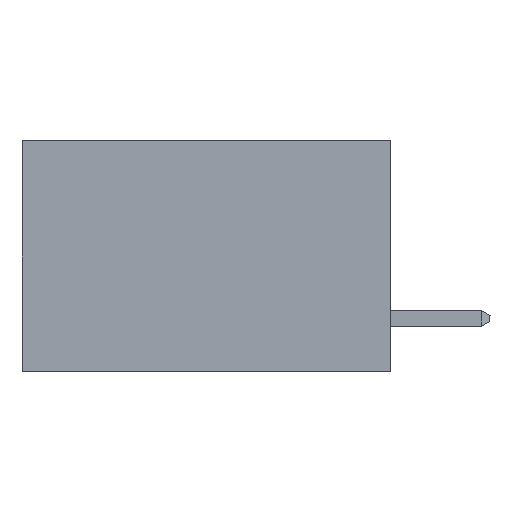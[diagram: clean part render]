
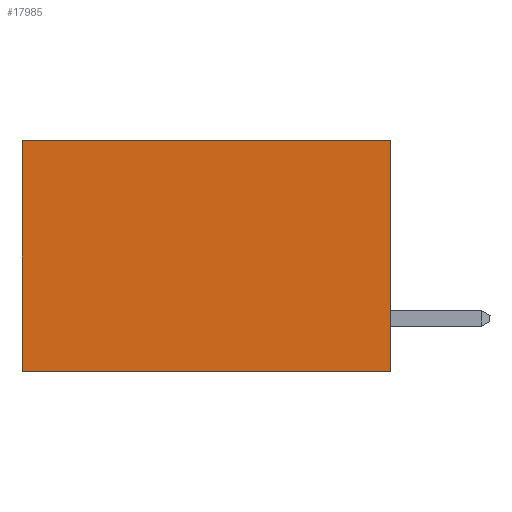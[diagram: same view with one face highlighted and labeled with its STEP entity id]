
A CAD part, left-side view. The second image highlights one B-rep face of the part: STEP entity #17985.
In plain terms, the highlighted planar face has unit normal (-1, 0, 0).
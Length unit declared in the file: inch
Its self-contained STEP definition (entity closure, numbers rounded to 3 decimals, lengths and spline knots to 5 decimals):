
#2036 = VERTEX_POINT ( 'NONE', #12464 ) ;
#2670 = EDGE_CURVE ( 'NONE', #18537, #3375, #8628, .T. ) ;
#3125 = AXIS2_PLACEMENT_3D ( 'NONE', #4354, #16279, #7392 ) ;
#3375 = VERTEX_POINT ( 'NONE', #13923 ) ;
#4354 = CARTESIAN_POINT ( 'NONE',  ( 0.277, 0., -0.37 ) ) ;
#4413 = PLANE ( 'NONE',  #3125 ) ;
#4489 = VERTEX_POINT ( 'NONE', #13480 ) ;
#4725 = DIRECTION ( 'NONE',  ( 0., 1., 0. ) ) ;
#4790 = VECTOR ( 'NONE', #13494, 39.37008 ) ;
#4847 = EDGE_CURVE ( 'NONE', #2036, #18537, #18902, .T. ) ;
#4871 = ORIENTED_EDGE ( 'NONE', *, *, #6501, .T. ) ;
#5317 = ORIENTED_EDGE ( 'NONE', *, *, #2670, .F. ) ;
#5808 = ORIENTED_EDGE ( 'NONE', *, *, #4847, .F. ) ;
#6067 = EDGE_LOOP ( 'NONE', ( #8196, #5317, #5808, #4871 ) ) ;
#6172 = LINE ( 'NONE', #13827, #4790 ) ;
#6501 = EDGE_CURVE ( 'NONE', #2036, #4489, #6172, .T. ) ;
#7392 = DIRECTION ( 'NONE',  ( 0., 0., -1. ) ) ;
#8167 = VECTOR ( 'NONE', #4725, 39.37008 ) ;
#8196 = ORIENTED_EDGE ( 'NONE', *, *, #14870, .T. ) ;
#8628 = LINE ( 'NONE', #17657, #8167 ) ;
#9698 = CARTESIAN_POINT ( 'NONE',  ( 0.277, 0., -0.37 ) ) ;
#9716 = DIRECTION ( 'NONE',  ( 0., 0., -1. ) ) ;
#10768 = FACE_OUTER_BOUND ( 'NONE', #6067, .T. ) ;
#11410 = VECTOR ( 'NONE', #9716, 39.37008 ) ;
#12464 = CARTESIAN_POINT ( 'NONE',  ( 0.277, 0., 0. ) ) ;
#12787 = VECTOR ( 'NONE', #17960, 39.37008 ) ;
#13095 = CARTESIAN_POINT ( 'NONE',  ( 0.277, 0., -0.37 ) ) ;
#13480 = CARTESIAN_POINT ( 'NONE',  ( 0.277, 0.59, 0. ) ) ;
#13494 = DIRECTION ( 'NONE',  ( 0., 1., 0. ) ) ;
#13827 = CARTESIAN_POINT ( 'NONE',  ( 0.277, 0., 0. ) ) ;
#13923 = CARTESIAN_POINT ( 'NONE',  ( 0.277, 0.59, -0.37 ) ) ;
#14870 = EDGE_CURVE ( 'NONE', #4489, #3375, #16684, .T. ) ;
#16279 = DIRECTION ( 'NONE',  ( 1., 0., 0. ) ) ;
#16593 = CARTESIAN_POINT ( 'NONE',  ( 0.277, 0.59, -0.37 ) ) ;
#16684 = LINE ( 'NONE', #16593, #12787 ) ;
#17657 = CARTESIAN_POINT ( 'NONE',  ( 0.277, 0., -0.37 ) ) ;
#17960 = DIRECTION ( 'NONE',  ( 0., 0., -1. ) ) ;
#17985 = ADVANCED_FACE ( 'NONE', ( #10768 ), #4413, .F. ) ;
#18537 = VERTEX_POINT ( 'NONE', #13095 ) ;
#18902 = LINE ( 'NONE', #9698, #11410 ) ;
